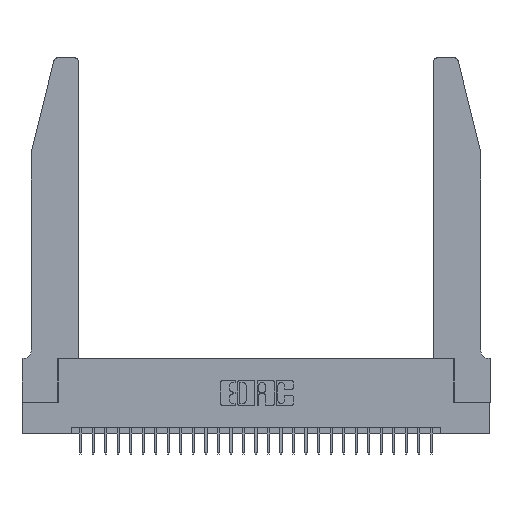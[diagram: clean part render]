
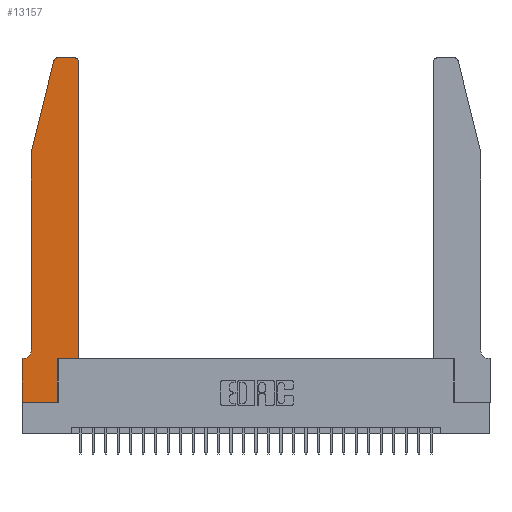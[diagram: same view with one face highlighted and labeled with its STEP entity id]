
A CAD part, top view. The second image highlights one B-rep face of the part: STEP entity #13157.
In plain terms, the highlighted planar face has unit normal (0, 0, 1).
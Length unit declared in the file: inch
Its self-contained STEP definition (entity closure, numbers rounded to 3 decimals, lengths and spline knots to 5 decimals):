
#282 = VERTEX_POINT ( 'NONE', #27928 ) ;
#653 = VERTEX_POINT ( 'NONE', #25826 ) ;
#993 = CARTESIAN_POINT ( 'NONE',  ( 0., 0., 0.37 ) ) ;
#1030 = CARTESIAN_POINT ( 'NONE',  ( 0.0755, 2., 0.37 ) ) ;
#1076 = CARTESIAN_POINT ( 'NONE',  ( 0.4205, 2.72, 0.37 ) ) ;
#1896 = ORIENTED_EDGE ( 'NONE', *, *, #15246, .T. ) ;
#2480 = DIRECTION ( 'NONE',  ( -1., 0., 0. ) ) ;
#2681 = DIRECTION ( 'NONE',  ( 1., 0., 0. ) ) ;
#2796 = VERTEX_POINT ( 'NONE', #23549 ) ;
#2917 = AXIS2_PLACEMENT_3D ( 'NONE', #22069, #8673, #24273 ) ;
#3381 = ORIENTED_EDGE ( 'NONE', *, *, #3977, .T. ) ;
#3443 = DIRECTION ( 'NONE',  ( 1., 0., 0. ) ) ;
#3504 = DIRECTION ( 'NONE',  ( 0., -1., 0. ) ) ;
#3682 = LINE ( 'NONE', #11841, #20377 ) ;
#3977 = EDGE_CURVE ( 'NONE', #22029, #7640, #12571, .T. ) ;
#4129 = LINE ( 'NONE', #9848, #8898 ) ;
#4430 = CIRCLE ( 'NONE', #18629, 0.07 ) ;
#5255 = VECTOR ( 'NONE', #21640, 39.37008 ) ;
#5475 = CIRCLE ( 'NONE', #18758, 0.03 ) ;
#5812 = CARTESIAN_POINT ( 'NONE',  ( 0.0755, 0.42, 0.37 ) ) ;
#6823 = DIRECTION ( 'NONE',  ( 0., 1., 0. ) ) ;
#7174 = VERTEX_POINT ( 'NONE', #5812 ) ;
#7311 = EDGE_LOOP ( 'NONE', ( #10280, #12423, #13825, #23206, #1896, #3381, #16993, #27762, #12105, #18705, #19425, #20816 ) ) ;
#7445 = EDGE_CURVE ( 'NONE', #25407, #19286, #19458, .T. ) ;
#7482 = EDGE_CURVE ( 'NONE', #19286, #25633, #12850, .T. ) ;
#7640 = VERTEX_POINT ( 'NONE', #24836 ) ;
#8021 = EDGE_CURVE ( 'NONE', #2796, #28433, #17360, .T. ) ;
#8221 = VECTOR ( 'NONE', #18181, 39.37008 ) ;
#8673 = DIRECTION ( 'NONE',  ( 0., 0., 1. ) ) ;
#8898 = VECTOR ( 'NONE', #23210, 39.37008 ) ;
#9645 = DIRECTION ( 'NONE',  ( 0., 0., -1. ) ) ;
#9848 = CARTESIAN_POINT ( 'NONE',  ( 0., 0., 0.37 ) ) ;
#10280 = ORIENTED_EDGE ( 'NONE', *, *, #8021, .T. ) ;
#10365 = DIRECTION ( 'NONE',  ( 1., 0., 0. ) ) ;
#11302 = EDGE_CURVE ( 'NONE', #15402, #2796, #5475, .T. ) ;
#11472 = EDGE_CURVE ( 'NONE', #28433, #282, #12669, .T. ) ;
#11841 = CARTESIAN_POINT ( 'NONE',  ( 0.0755, 2., 0.37 ) ) ;
#11864 = VECTOR ( 'NONE', #2480, 39.37008 ) ;
#11868 = CARTESIAN_POINT ( 'NONE',  ( 0.284, 2.75, 0.37 ) ) ;
#12105 = ORIENTED_EDGE ( 'NONE', *, *, #7482, .T. ) ;
#12423 = ORIENTED_EDGE ( 'NONE', *, *, #11472, .T. ) ;
#12529 = CARTESIAN_POINT ( 'NONE',  ( 0.2865, 0., 0.37 ) ) ;
#12571 = LINE ( 'NONE', #18450, #11864 ) ;
#12669 = CIRCLE ( 'NONE', #2917, 0.03 ) ;
#12821 = FACE_OUTER_BOUND ( 'NONE', #7311, .T. ) ;
#12850 = LINE ( 'NONE', #22737, #23950 ) ;
#13157 = ADVANCED_FACE ( 'NONE', ( #12821 ), #17042, .T. ) ;
#13825 = ORIENTED_EDGE ( 'NONE', *, *, #24556, .T. ) ;
#14086 = DIRECTION ( 'NONE',  ( -0.239, -0.971, 0. ) ) ;
#14186 = CARTESIAN_POINT ( 'NONE',  ( 0.4505, 0.35, 0.37 ) ) ;
#15246 = EDGE_CURVE ( 'NONE', #7174, #22029, #4430, .T. ) ;
#15262 = EDGE_CURVE ( 'NONE', #25633, #16703, #21083, .T. ) ;
#15402 = VERTEX_POINT ( 'NONE', #21355 ) ;
#15480 = EDGE_CURVE ( 'NONE', #653, #7174, #28017, .T. ) ;
#15953 = CARTESIAN_POINT ( 'NONE',  ( 0., 0., 0.37 ) ) ;
#16051 = LINE ( 'NONE', #18085, #27175 ) ;
#16703 = VERTEX_POINT ( 'NONE', #21933 ) ;
#16993 = ORIENTED_EDGE ( 'NONE', *, *, #23441, .T. ) ;
#17042 = PLANE ( 'NONE',  #26435 ) ;
#17141 = DIRECTION ( 'NONE',  ( 0., 0., 1. ) ) ;
#17360 = LINE ( 'NONE', #28328, #5255 ) ;
#18032 = EDGE_CURVE ( 'NONE', #16703, #15402, #16051, .T. ) ;
#18085 = CARTESIAN_POINT ( 'NONE',  ( 0.4505, 0.35, 0.37 ) ) ;
#18181 = DIRECTION ( 'NONE',  ( 1., 0., 0. ) ) ;
#18450 = CARTESIAN_POINT ( 'NONE',  ( 0.0755, 0.35, 0.37 ) ) ;
#18629 = AXIS2_PLACEMENT_3D ( 'NONE', #23016, #9645, #25226 ) ;
#18705 = ORIENTED_EDGE ( 'NONE', *, *, #15262, .T. ) ;
#18758 = AXIS2_PLACEMENT_3D ( 'NONE', #1076, #17141, #3443 ) ;
#19286 = VERTEX_POINT ( 'NONE', #12529 ) ;
#19425 = ORIENTED_EDGE ( 'NONE', *, *, #18032, .T. ) ;
#19458 = LINE ( 'NONE', #15953, #8221 ) ;
#20038 = CARTESIAN_POINT ( 'NONE',  ( 0.2865, 0.35, 0.37 ) ) ;
#20377 = VECTOR ( 'NONE', #14086, 39.37008 ) ;
#20722 = VECTOR ( 'NONE', #3504, 39.37008 ) ;
#20816 = ORIENTED_EDGE ( 'NONE', *, *, #11302, .T. ) ;
#21083 = LINE ( 'NONE', #14186, #27008 ) ;
#21355 = CARTESIAN_POINT ( 'NONE',  ( 0.4505, 2.72, 0.37 ) ) ;
#21486 = CARTESIAN_POINT ( 'NONE',  ( 0., 0.35, 0.37 ) ) ;
#21640 = DIRECTION ( 'NONE',  ( -1., 0., 0. ) ) ;
#21933 = CARTESIAN_POINT ( 'NONE',  ( 0.4505, 0.35, 0.37 ) ) ;
#22029 = VERTEX_POINT ( 'NONE', #24526 ) ;
#22069 = CARTESIAN_POINT ( 'NONE',  ( 0.284, 2.72, 0.37 ) ) ;
#22737 = CARTESIAN_POINT ( 'NONE',  ( 0.2865, 0.35, 0.37 ) ) ;
#23016 = CARTESIAN_POINT ( 'NONE',  ( 0.0055, 0.42, 0.37 ) ) ;
#23206 = ORIENTED_EDGE ( 'NONE', *, *, #15480, .T. ) ;
#23210 = DIRECTION ( 'NONE',  ( 0., -1., 0. ) ) ;
#23441 = EDGE_CURVE ( 'NONE', #7640, #25407, #4129, .T. ) ;
#23549 = CARTESIAN_POINT ( 'NONE',  ( 0.4205, 2.75, 0.37 ) ) ;
#23700 = DIRECTION ( 'NONE',  ( 0., 0., 1. ) ) ;
#23950 = VECTOR ( 'NONE', #24950, 39.37008 ) ;
#24273 = DIRECTION ( 'NONE',  ( 1., 0., 0. ) ) ;
#24526 = CARTESIAN_POINT ( 'NONE',  ( 0.0055, 0.35, 0.37 ) ) ;
#24556 = EDGE_CURVE ( 'NONE', #282, #653, #3682, .T. ) ;
#24836 = CARTESIAN_POINT ( 'NONE',  ( 0., 0.35, 0.37 ) ) ;
#24950 = DIRECTION ( 'NONE',  ( 0., 1., 0. ) ) ;
#25226 = DIRECTION ( 'NONE',  ( -1., 0., 0. ) ) ;
#25407 = VERTEX_POINT ( 'NONE', #993 ) ;
#25633 = VERTEX_POINT ( 'NONE', #20038 ) ;
#25826 = CARTESIAN_POINT ( 'NONE',  ( 0.0755, 2., 0.37 ) ) ;
#26435 = AXIS2_PLACEMENT_3D ( 'NONE', #21486, #23700, #10365 ) ;
#27008 = VECTOR ( 'NONE', #2681, 39.37008 ) ;
#27175 = VECTOR ( 'NONE', #6823, 39.37008 ) ;
#27762 = ORIENTED_EDGE ( 'NONE', *, *, #7445, .T. ) ;
#27928 = CARTESIAN_POINT ( 'NONE',  ( 0.25487, 2.72718, 0.37 ) ) ;
#28017 = LINE ( 'NONE', #1030, #20722 ) ;
#28328 = CARTESIAN_POINT ( 'NONE',  ( 0.2605, 2.75, 0.37 ) ) ;
#28433 = VERTEX_POINT ( 'NONE', #11868 ) ;
